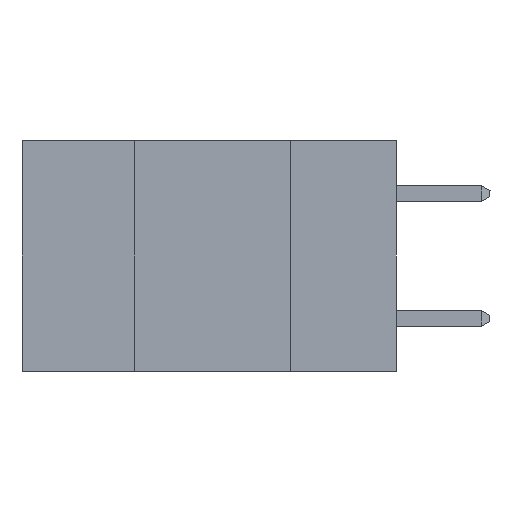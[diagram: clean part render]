
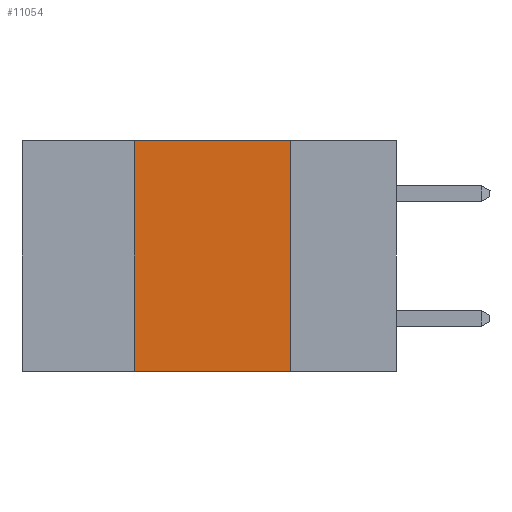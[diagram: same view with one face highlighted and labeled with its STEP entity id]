
A CAD part, left-side view. The second image highlights one B-rep face of the part: STEP entity #11054.
In plain terms, the highlighted planar face has unit normal (-1, 0, 0).
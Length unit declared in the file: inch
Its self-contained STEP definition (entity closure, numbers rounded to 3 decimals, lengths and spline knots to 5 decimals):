
#325 = LINE ( 'NONE', #3068, #5788 ) ;
#648 = VERTEX_POINT ( 'NONE', #1399 ) ;
#1156 = VERTEX_POINT ( 'NONE', #6011 ) ;
#1198 = CARTESIAN_POINT ( 'NONE',  ( 0., 0.6, 0. ) ) ;
#1357 = VECTOR ( 'NONE', #9002, 39.37008 ) ;
#1399 = CARTESIAN_POINT ( 'NONE',  ( 0., 0.42, -0.37 ) ) ;
#1702 = LINE ( 'NONE', #9061, #1357 ) ;
#2296 = PLANE ( 'NONE',  #12106 ) ;
#2430 = EDGE_CURVE ( 'NONE', #648, #7397, #325, .T. ) ;
#2889 = ORIENTED_EDGE ( 'NONE', *, *, #3245, .F. ) ;
#3068 = CARTESIAN_POINT ( 'NONE',  ( 0., 0.42, 0. ) ) ;
#3245 = EDGE_CURVE ( 'NONE', #7397, #4638, #1702, .T. ) ;
#3369 = DIRECTION ( 'NONE',  ( 0., 0., 1. ) ) ;
#3883 = DIRECTION ( 'NONE',  ( 0., -1., 0. ) ) ;
#4159 = CARTESIAN_POINT ( 'NONE',  ( 0., 0.17, 0. ) ) ;
#4177 = ORIENTED_EDGE ( 'NONE', *, *, #6797, .F. ) ;
#4463 = DIRECTION ( 'NONE',  ( 1., 0., 0. ) ) ;
#4638 = VERTEX_POINT ( 'NONE', #6789 ) ;
#4842 = VECTOR ( 'NONE', #5225, 39.37008 ) ;
#5225 = DIRECTION ( 'NONE',  ( 0., 0., -1. ) ) ;
#5788 = VECTOR ( 'NONE', #3369, 39.37008 ) ;
#6011 = CARTESIAN_POINT ( 'NONE',  ( 0., 0.17, -0.37 ) ) ;
#6789 = CARTESIAN_POINT ( 'NONE',  ( 0., 0.17, 0. ) ) ;
#6797 = EDGE_CURVE ( 'NONE', #4638, #1156, #13275, .T. ) ;
#7190 = FACE_OUTER_BOUND ( 'NONE', #11183, .T. ) ;
#7397 = VERTEX_POINT ( 'NONE', #12487 ) ;
#7946 = ORIENTED_EDGE ( 'NONE', *, *, #2430, .F. ) ;
#9002 = DIRECTION ( 'NONE',  ( 0., -1., 0. ) ) ;
#9049 = ORIENTED_EDGE ( 'NONE', *, *, #9694, .T. ) ;
#9061 = CARTESIAN_POINT ( 'NONE',  ( 0., 0.6, 0. ) ) ;
#9694 = EDGE_CURVE ( 'NONE', #648, #1156, #13539, .T. ) ;
#9793 = DIRECTION ( 'NONE',  ( 0., 0., -1. ) ) ;
#10236 = CARTESIAN_POINT ( 'NONE',  ( 0., 0.6, -0.37 ) ) ;
#10393 = VECTOR ( 'NONE', #3883, 39.37008 ) ;
#11054 = ADVANCED_FACE ( 'NONE', ( #7190 ), #2296, .F. ) ;
#11183 = EDGE_LOOP ( 'NONE', ( #4177, #2889, #7946, #9049 ) ) ;
#12106 = AXIS2_PLACEMENT_3D ( 'NONE', #1198, #4463, #9793 ) ;
#12487 = CARTESIAN_POINT ( 'NONE',  ( 0., 0.42, 0. ) ) ;
#13275 = LINE ( 'NONE', #4159, #4842 ) ;
#13539 = LINE ( 'NONE', #10236, #10393 ) ;
